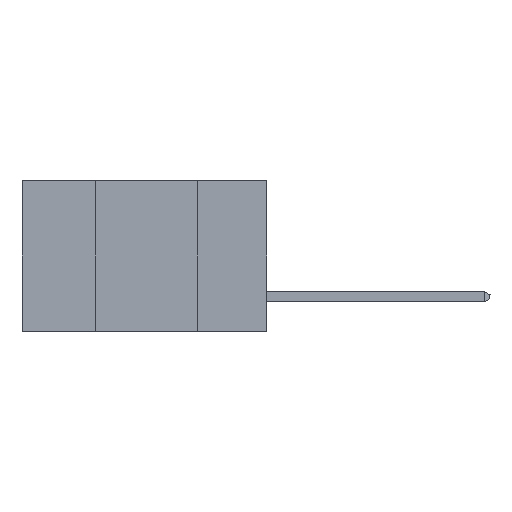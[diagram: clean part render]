
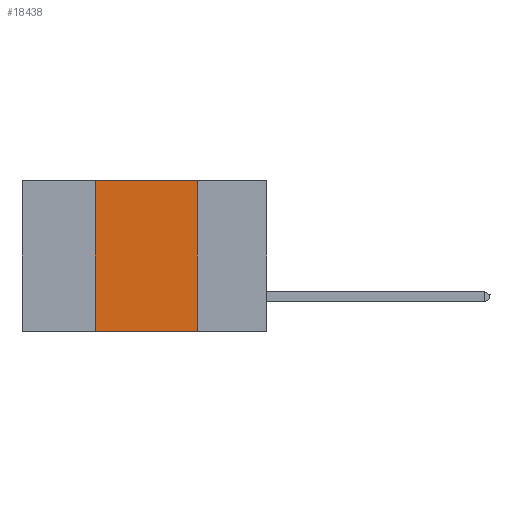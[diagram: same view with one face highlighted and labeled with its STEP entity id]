
A CAD part, left-side view. The second image highlights one B-rep face of the part: STEP entity #18438.
In plain terms, the highlighted planar face has unit normal (-1, 0, 0).
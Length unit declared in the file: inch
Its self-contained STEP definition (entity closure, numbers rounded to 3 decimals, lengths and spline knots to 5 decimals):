
#90 = EDGE_LOOP ( 'NONE', ( #16046, #4699, #15868, #1517 ) ) ;
#496 = VERTEX_POINT ( 'NONE', #17533 ) ;
#1144 = LINE ( 'NONE', #11988, #7933 ) ;
#1507 = EDGE_CURVE ( 'NONE', #8225, #3788, #5927, .T. ) ;
#1517 = ORIENTED_EDGE ( 'NONE', *, *, #9136, .T. ) ;
#3303 = DIRECTION ( 'NONE',  ( 0., 0., -1. ) ) ;
#3359 = CARTESIAN_POINT ( 'NONE',  ( 0., 0.17, 0. ) ) ;
#3788 = VERTEX_POINT ( 'NONE', #6034 ) ;
#4183 = DIRECTION ( 'NONE',  ( 0., -1., 0. ) ) ;
#4233 = DIRECTION ( 'NONE',  ( 0., 0., -1. ) ) ;
#4687 = FACE_OUTER_BOUND ( 'NONE', #90, .T. ) ;
#4699 = ORIENTED_EDGE ( 'NONE', *, *, #19482, .F. ) ;
#5927 = LINE ( 'NONE', #7350, #7277 ) ;
#6034 = CARTESIAN_POINT ( 'NONE',  ( 0., 0.17, -0.37 ) ) ;
#6881 = DIRECTION ( 'NONE',  ( 1., 0., 0. ) ) ;
#6896 = VERTEX_POINT ( 'NONE', #17083 ) ;
#7252 = DIRECTION ( 'NONE',  ( 0., 0., 1. ) ) ;
#7277 = VECTOR ( 'NONE', #4233, 39.37008 ) ;
#7350 = CARTESIAN_POINT ( 'NONE',  ( 0., 0.17, 0. ) ) ;
#7486 = LINE ( 'NONE', #10502, #10384 ) ;
#7933 = VECTOR ( 'NONE', #7252, 39.37008 ) ;
#8225 = VERTEX_POINT ( 'NONE', #3359 ) ;
#9136 = EDGE_CURVE ( 'NONE', #496, #3788, #16034, .T. ) ;
#10384 = VECTOR ( 'NONE', #4183, 39.37008 ) ;
#10502 = CARTESIAN_POINT ( 'NONE',  ( 0., 0.6, 0. ) ) ;
#10824 = CARTESIAN_POINT ( 'NONE',  ( 0., 0.6, 0. ) ) ;
#11224 = DIRECTION ( 'NONE',  ( 0., -1., 0. ) ) ;
#11988 = CARTESIAN_POINT ( 'NONE',  ( 0., 0.42, 0. ) ) ;
#12598 = VECTOR ( 'NONE', #11224, 39.37008 ) ;
#13777 = EDGE_CURVE ( 'NONE', #496, #6896, #1144, .T. ) ;
#15868 = ORIENTED_EDGE ( 'NONE', *, *, #13777, .F. ) ;
#16034 = LINE ( 'NONE', #19028, #12598 ) ;
#16046 = ORIENTED_EDGE ( 'NONE', *, *, #1507, .F. ) ;
#17083 = CARTESIAN_POINT ( 'NONE',  ( 0., 0.42, 0. ) ) ;
#17150 = PLANE ( 'NONE',  #19317 ) ;
#17533 = CARTESIAN_POINT ( 'NONE',  ( 0., 0.42, -0.37 ) ) ;
#18438 = ADVANCED_FACE ( 'NONE', ( #4687 ), #17150, .F. ) ;
#19028 = CARTESIAN_POINT ( 'NONE',  ( 0., 0.6, -0.37 ) ) ;
#19317 = AXIS2_PLACEMENT_3D ( 'NONE', #10824, #6881, #3303 ) ;
#19482 = EDGE_CURVE ( 'NONE', #6896, #8225, #7486, .T. ) ;
